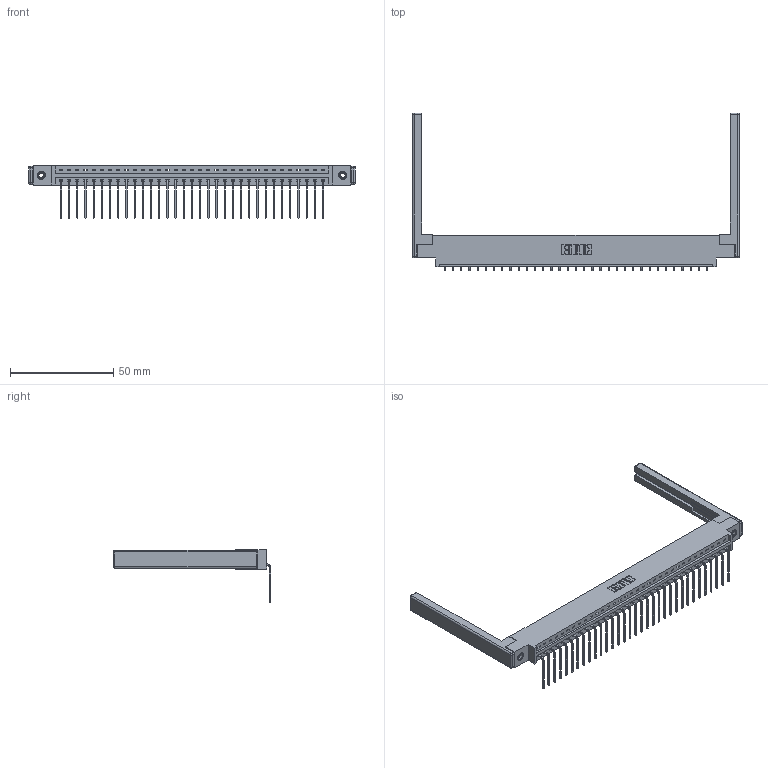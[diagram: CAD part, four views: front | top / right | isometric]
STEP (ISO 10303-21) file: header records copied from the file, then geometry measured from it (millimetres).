
FILE_DESCRIPTION (( 'STEP AP203' ), '1' );
FILE_NAME ('337-033-559-668.STEP', '2019-10-01T11:14:03', ( '' ), ( '' ), 'SwSTEP 2.0', 'SolidWorks 2016', '' );
FILE_SCHEMA (( 'CONFIG_CONTROL_DESIGN' ));
Length unit declared in the file: inch
Products named in the file (5): 307-220-068; 337-033-559-668; 337 Part_0.170 Offset - 0.156 Dia-TI; 345-292-001_558 559 Tail - 1; 345-250-001_345-250-001-102
Assembly tree (38 placements, depth 2):
  337-033-559-668
    337 Part_0.170 Offset - 0.156 Dia-TI
    345-292-001_558 559 Tail - 1  x33
    345-250-001_345-250-001-102  x2
    307-220-068  x2
Bounding box: 158.19 x 76.14 x 25.53 mm (x, y, z)
Volume: 20712.4 mm3; surface area: 21680.1 mm2
Topology: 38 solids, 38 shells, 2384 faces, 7115 edges, 4678 vertices
Faces by surface type: plane 1746, cylinder 614, cone 12, sphere 8, torus 4
Entity records: 28670 total; most frequent: CARTESIAN_POINT 4950, ORIENTED_EDGE 4908, DIRECTION 4258, EDGE_CURVE 2454, LINE 2276, VECTOR 2276, VERTEX_POINT 1626, AXIS2_PLACEMENT_3D 991
